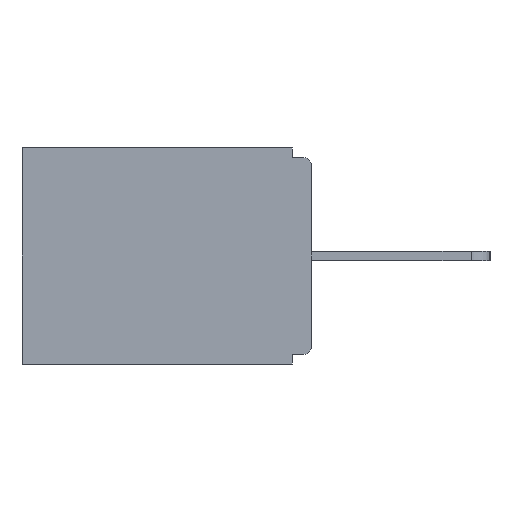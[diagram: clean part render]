
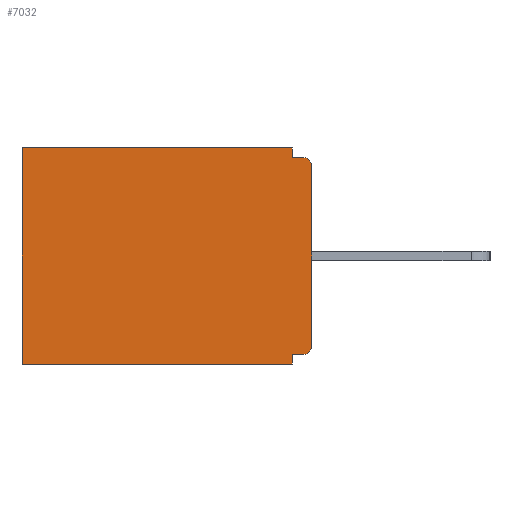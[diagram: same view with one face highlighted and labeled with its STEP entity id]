
A CAD part, left-side view. The second image highlights one B-rep face of the part: STEP entity #7032.
In plain terms, the highlighted planar face has unit normal (-1, 0, 0).
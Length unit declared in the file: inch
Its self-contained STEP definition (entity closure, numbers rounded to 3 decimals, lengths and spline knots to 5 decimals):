
#139 = CARTESIAN_POINT ( 'NONE',  ( 0.298, 0., -0.015 ) ) ;
#340 = CARTESIAN_POINT ( 'NONE',  ( 0.298, 0.015, -0.313 ) ) ;
#462 = AXIS2_PLACEMENT_3D ( 'NONE', #340, #4369, #5867 ) ;
#919 = VECTOR ( 'NONE', #8899, 39.37008 ) ;
#1146 = LINE ( 'NONE', #17052, #7440 ) ;
#1394 = VERTEX_POINT ( 'NONE', #4070 ) ;
#2271 = EDGE_CURVE ( 'NONE', #15951, #8859, #5768, .T. ) ;
#2332 = LINE ( 'NONE', #7678, #13132 ) ;
#2385 = ORIENTED_EDGE ( 'NONE', *, *, #2271, .F. ) ;
#3177 = VECTOR ( 'NONE', #8325, 39.37008 ) ;
#3242 = EDGE_CURVE ( 'NONE', #8859, #11704, #1146, .T. ) ;
#3350 = CARTESIAN_POINT ( 'NONE',  ( 0.298, 0.46, -0.343 ) ) ;
#3466 = DIRECTION ( 'NONE',  ( 0., 0., -1. ) ) ;
#3497 = DIRECTION ( 'NONE',  ( -1., 0., 0. ) ) ;
#3540 = CARTESIAN_POINT ( 'NONE',  ( 0.298, 0.031, -0.343 ) ) ;
#3792 = LINE ( 'NONE', #9755, #8346 ) ;
#3952 = VERTEX_POINT ( 'NONE', #13828 ) ;
#4070 = CARTESIAN_POINT ( 'NONE',  ( 0.298, 0., -0.03 ) ) ;
#4212 = LINE ( 'NONE', #10905, #10169 ) ;
#4232 = CARTESIAN_POINT ( 'NONE',  ( 0.298, 0.031, 0. ) ) ;
#4369 = DIRECTION ( 'NONE',  ( -1., 0., 0. ) ) ;
#4554 = EDGE_CURVE ( 'NONE', #5630, #3952, #15584, .T. ) ;
#4647 = VECTOR ( 'NONE', #15977, 39.37008 ) ;
#4690 = DIRECTION ( 'NONE',  ( 1., 0., 0. ) ) ;
#4847 = EDGE_CURVE ( 'NONE', #13599, #15951, #4212, .T. ) ;
#4915 = EDGE_CURVE ( 'NONE', #13599, #10647, #4946, .T. ) ;
#4946 = CIRCLE ( 'NONE', #462, 0.015 ) ;
#5079 = ORIENTED_EDGE ( 'NONE', *, *, #4847, .F. ) ;
#5142 = ORIENTED_EDGE ( 'NONE', *, *, #12251, .T. ) ;
#5183 = CARTESIAN_POINT ( 'NONE',  ( 0.298, 0.015, -0.328 ) ) ;
#5630 = VERTEX_POINT ( 'NONE', #4232 ) ;
#5768 = LINE ( 'NONE', #13671, #3177 ) ;
#5867 = DIRECTION ( 'NONE',  ( 0., 0., -1. ) ) ;
#6031 = EDGE_CURVE ( 'NONE', #1394, #10647, #3792, .T. ) ;
#6364 = CIRCLE ( 'NONE', #17033, 0.015 ) ;
#6820 = EDGE_CURVE ( 'NONE', #12142, #11704, #17362, .T. ) ;
#6932 = DIRECTION ( 'NONE',  ( 0., 1., 0. ) ) ;
#7023 = DIRECTION ( 'NONE',  ( 0., 0., -1. ) ) ;
#7032 = ADVANCED_FACE ( 'NONE', ( #15421 ), #11471, .F. ) ;
#7143 = CARTESIAN_POINT ( 'NONE',  ( 0.298, 0.015, -0.015 ) ) ;
#7440 = VECTOR ( 'NONE', #14145, 39.37008 ) ;
#7678 = CARTESIAN_POINT ( 'NONE',  ( 0.298, 0., 0. ) ) ;
#7755 = EDGE_LOOP ( 'NONE', ( #5142, #8146, #13334, #16845, #8928, #16159, #2385, #5079, #17299, #14898 ) ) ;
#8146 = ORIENTED_EDGE ( 'NONE', *, *, #11116, .F. ) ;
#8325 = DIRECTION ( 'NONE',  ( 0., 0., -1. ) ) ;
#8346 = VECTOR ( 'NONE', #7023, 39.37008 ) ;
#8859 = VERTEX_POINT ( 'NONE', #14336 ) ;
#8899 = DIRECTION ( 'NONE',  ( 0., 0., -1. ) ) ;
#8906 = CARTESIAN_POINT ( 'NONE',  ( 0.298, 0., 0. ) ) ;
#8928 = ORIENTED_EDGE ( 'NONE', *, *, #6820, .T. ) ;
#9573 = CARTESIAN_POINT ( 'NONE',  ( 0.298, 0., -0.313 ) ) ;
#9755 = CARTESIAN_POINT ( 'NONE',  ( 0.298, 0., 0. ) ) ;
#10169 = VECTOR ( 'NONE', #6932, 39.37008 ) ;
#10647 = VERTEX_POINT ( 'NONE', #9573 ) ;
#10905 = CARTESIAN_POINT ( 'NONE',  ( 0.298, 0., -0.328 ) ) ;
#11116 = EDGE_CURVE ( 'NONE', #3952, #12947, #17287, .T. ) ;
#11471 = PLANE ( 'NONE',  #13728 ) ;
#11704 = VERTEX_POINT ( 'NONE', #3350 ) ;
#11760 = DIRECTION ( 'NONE',  ( 0., 0., -1. ) ) ;
#11832 = DIRECTION ( 'NONE',  ( 0., 0., -1. ) ) ;
#12008 = CARTESIAN_POINT ( 'NONE',  ( 0.298, 0.46, 0. ) ) ;
#12087 = VECTOR ( 'NONE', #11832, 39.37008 ) ;
#12142 = VERTEX_POINT ( 'NONE', #16508 ) ;
#12251 = EDGE_CURVE ( 'NONE', #1394, #12947, #6364, .T. ) ;
#12895 = CARTESIAN_POINT ( 'NONE',  ( 0.298, 0.015, -0.03 ) ) ;
#12947 = VERTEX_POINT ( 'NONE', #7143 ) ;
#12962 = DIRECTION ( 'NONE',  ( 0., 1., 0. ) ) ;
#13132 = VECTOR ( 'NONE', #12962, 39.37008 ) ;
#13188 = CARTESIAN_POINT ( 'NONE',  ( 0.298, 0.031, -0.328 ) ) ;
#13334 = ORIENTED_EDGE ( 'NONE', *, *, #4554, .F. ) ;
#13599 = VERTEX_POINT ( 'NONE', #5183 ) ;
#13671 = CARTESIAN_POINT ( 'NONE',  ( 0.298, 0.031, -0.343 ) ) ;
#13728 = AXIS2_PLACEMENT_3D ( 'NONE', #8906, #4690, #3466 ) ;
#13828 = CARTESIAN_POINT ( 'NONE',  ( 0.298, 0.031, -0.015 ) ) ;
#14145 = DIRECTION ( 'NONE',  ( 0., 1., 0. ) ) ;
#14336 = CARTESIAN_POINT ( 'NONE',  ( 0.298, 0.031, -0.343 ) ) ;
#14898 = ORIENTED_EDGE ( 'NONE', *, *, #6031, .F. ) ;
#15421 = FACE_OUTER_BOUND ( 'NONE', #7755, .T. ) ;
#15584 = LINE ( 'NONE', #3540, #919 ) ;
#15951 = VERTEX_POINT ( 'NONE', #13188 ) ;
#15977 = DIRECTION ( 'NONE',  ( 0., -1., 0. ) ) ;
#16159 = ORIENTED_EDGE ( 'NONE', *, *, #3242, .F. ) ;
#16508 = CARTESIAN_POINT ( 'NONE',  ( 0.298, 0.46, 0. ) ) ;
#16656 = EDGE_CURVE ( 'NONE', #5630, #12142, #2332, .T. ) ;
#16845 = ORIENTED_EDGE ( 'NONE', *, *, #16656, .T. ) ;
#17033 = AXIS2_PLACEMENT_3D ( 'NONE', #12895, #3497, #11760 ) ;
#17052 = CARTESIAN_POINT ( 'NONE',  ( 0.298, 0., -0.343 ) ) ;
#17287 = LINE ( 'NONE', #139, #4647 ) ;
#17299 = ORIENTED_EDGE ( 'NONE', *, *, #4915, .T. ) ;
#17362 = LINE ( 'NONE', #12008, #12087 ) ;
